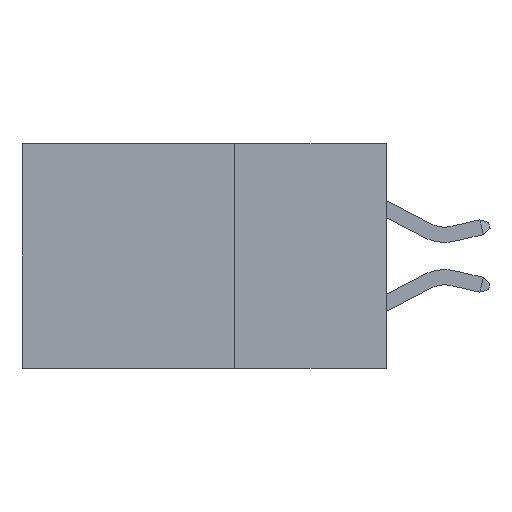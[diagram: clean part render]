
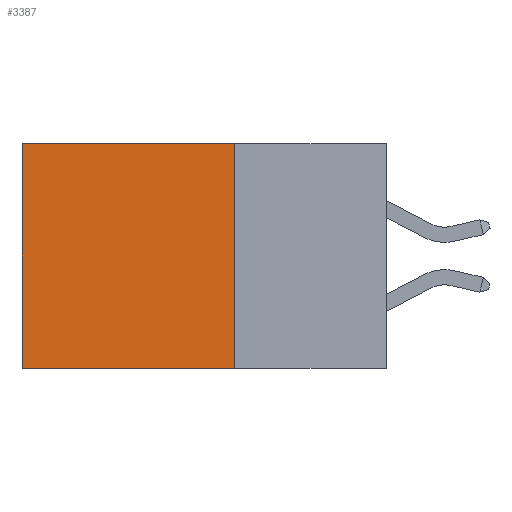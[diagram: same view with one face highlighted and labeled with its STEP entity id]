
A CAD part, left-side view. The second image highlights one B-rep face of the part: STEP entity #3387.
In plain terms, the highlighted planar face has unit normal (-1, 0, 0).
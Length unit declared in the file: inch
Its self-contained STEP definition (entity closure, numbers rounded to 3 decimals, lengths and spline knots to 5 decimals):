
#364 = CARTESIAN_POINT ( 'NONE',  ( 0.298, 0.6, 0. ) ) ;
#402 = CARTESIAN_POINT ( 'NONE',  ( 0.298, 0.25, 0. ) ) ;
#742 = VERTEX_POINT ( 'NONE', #364 ) ;
#2128 = DIRECTION ( 'NONE',  ( 1., 0., 0. ) ) ;
#2420 = AXIS2_PLACEMENT_3D ( 'NONE', #29379, #2128, #18100 ) ;
#2522 = EDGE_CURVE ( 'NONE', #18205, #18838, #9254, .T. ) ;
#2686 = VECTOR ( 'NONE', #28854, 39.37008 ) ;
#3387 = ADVANCED_FACE ( 'NONE', ( #27937 ), #13598, .F. ) ;
#3944 = EDGE_CURVE ( 'NONE', #18838, #12851, #20905, .T. ) ;
#4143 = CARTESIAN_POINT ( 'NONE',  ( 0.298, 0.25, 0. ) ) ;
#4641 = CARTESIAN_POINT ( 'NONE',  ( 0.298, 0.6, -0.37 ) ) ;
#7376 = CARTESIAN_POINT ( 'NONE',  ( 0.298, 0.25, -0.37 ) ) ;
#9254 = LINE ( 'NONE', #402, #15305 ) ;
#9335 = EDGE_LOOP ( 'NONE', ( #18530, #12340, #21013, #10450 ) ) ;
#9531 = VECTOR ( 'NONE', #14157, 39.37008 ) ;
#9708 = EDGE_CURVE ( 'NONE', #742, #12851, #27553, .T. ) ;
#10450 = ORIENTED_EDGE ( 'NONE', *, *, #12730, .T. ) ;
#12340 = ORIENTED_EDGE ( 'NONE', *, *, #3944, .F. ) ;
#12730 = EDGE_CURVE ( 'NONE', #18205, #742, #14473, .T. ) ;
#12851 = VERTEX_POINT ( 'NONE', #4641 ) ;
#13598 = PLANE ( 'NONE',  #2420 ) ;
#14157 = DIRECTION ( 'NONE',  ( 0., 0., -1. ) ) ;
#14473 = LINE ( 'NONE', #4143, #25080 ) ;
#15305 = VECTOR ( 'NONE', #21676, 39.37008 ) ;
#15358 = CARTESIAN_POINT ( 'NONE',  ( 0.298, 0.25, -0.37 ) ) ;
#17797 = DIRECTION ( 'NONE',  ( 0., 1., 0. ) ) ;
#18100 = DIRECTION ( 'NONE',  ( 0., 0., -1. ) ) ;
#18205 = VERTEX_POINT ( 'NONE', #25326 ) ;
#18530 = ORIENTED_EDGE ( 'NONE', *, *, #9708, .T. ) ;
#18838 = VERTEX_POINT ( 'NONE', #7376 ) ;
#20905 = LINE ( 'NONE', #15358, #2686 ) ;
#21013 = ORIENTED_EDGE ( 'NONE', *, *, #2522, .F. ) ;
#21676 = DIRECTION ( 'NONE',  ( 0., 0., -1. ) ) ;
#25080 = VECTOR ( 'NONE', #17797, 39.37008 ) ;
#25326 = CARTESIAN_POINT ( 'NONE',  ( 0.298, 0.25, 0. ) ) ;
#25411 = CARTESIAN_POINT ( 'NONE',  ( 0.298, 0.6, 0. ) ) ;
#27553 = LINE ( 'NONE', #25411, #9531 ) ;
#27937 = FACE_OUTER_BOUND ( 'NONE', #9335, .T. ) ;
#28854 = DIRECTION ( 'NONE',  ( 0., 1., 0. ) ) ;
#29379 = CARTESIAN_POINT ( 'NONE',  ( 0.298, 0.25, 0. ) ) ;
